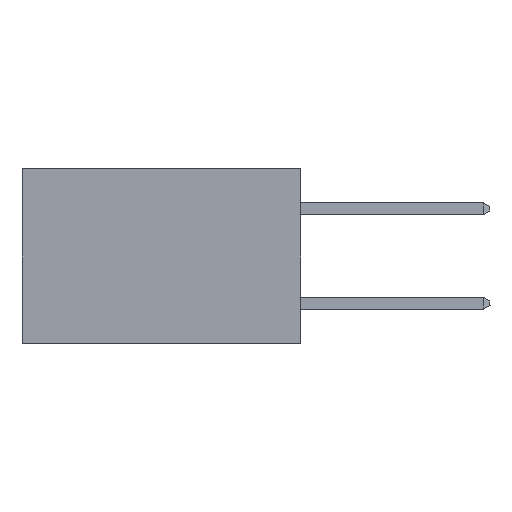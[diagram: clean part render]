
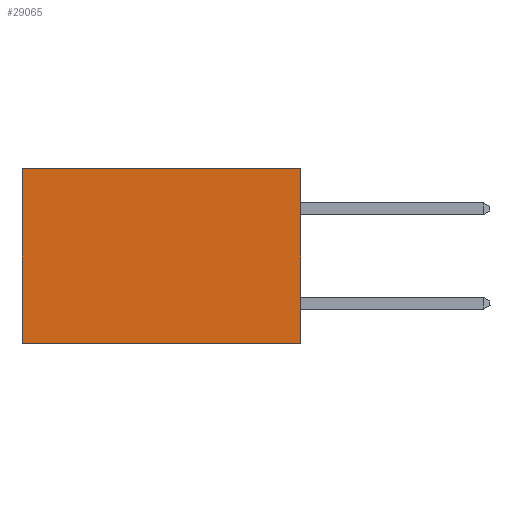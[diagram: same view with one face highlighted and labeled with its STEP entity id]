
A CAD part, left-side view. The second image highlights one B-rep face of the part: STEP entity #29065.
In plain terms, the highlighted planar face has unit normal (-1, 0, 0).
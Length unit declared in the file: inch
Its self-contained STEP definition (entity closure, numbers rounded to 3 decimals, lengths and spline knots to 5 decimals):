
#489 = EDGE_CURVE ( 'NONE', #24330, #6889, #16269, .T. ) ;
#1101 = CARTESIAN_POINT ( 'NONE',  ( 0.277, 0., -0.37 ) ) ;
#1385 = VECTOR ( 'NONE', #24439, 39.37008 ) ;
#2097 = EDGE_CURVE ( 'NONE', #6889, #4923, #13634, .T. ) ;
#4361 = ORIENTED_EDGE ( 'NONE', *, *, #17349, .T. ) ;
#4923 = VERTEX_POINT ( 'NONE', #20999 ) ;
#5316 = DIRECTION ( 'NONE',  ( 0., 1., 0. ) ) ;
#5651 = CARTESIAN_POINT ( 'NONE',  ( 0.277, 0., 0. ) ) ;
#6889 = VERTEX_POINT ( 'NONE', #11292 ) ;
#7578 = FACE_OUTER_BOUND ( 'NONE', #15338, .T. ) ;
#7612 = CARTESIAN_POINT ( 'NONE',  ( 0.277, 0., 0. ) ) ;
#8781 = VECTOR ( 'NONE', #11978, 39.37008 ) ;
#9785 = ORIENTED_EDGE ( 'NONE', *, *, #489, .F. ) ;
#10196 = VECTOR ( 'NONE', #17906, 39.37008 ) ;
#10547 = VERTEX_POINT ( 'NONE', #25921 ) ;
#11292 = CARTESIAN_POINT ( 'NONE',  ( 0.277, 0., -0.37 ) ) ;
#11978 = DIRECTION ( 'NONE',  ( 0., 0., -1. ) ) ;
#12576 = CARTESIAN_POINT ( 'NONE',  ( 0.277, 0., -0.37 ) ) ;
#13634 = LINE ( 'NONE', #12576, #1385 ) ;
#13737 = DIRECTION ( 'NONE',  ( 1., 0., 0. ) ) ;
#13950 = ORIENTED_EDGE ( 'NONE', *, *, #27455, .T. ) ;
#14354 = LINE ( 'NONE', #7612, #25838 ) ;
#14893 = LINE ( 'NONE', #23415, #8781 ) ;
#15338 = EDGE_LOOP ( 'NONE', ( #13950, #27346, #9785, #4361 ) ) ;
#16269 = LINE ( 'NONE', #1101, #10196 ) ;
#17349 = EDGE_CURVE ( 'NONE', #24330, #10547, #14354, .T. ) ;
#17906 = DIRECTION ( 'NONE',  ( 0., 0., -1. ) ) ;
#20581 = CARTESIAN_POINT ( 'NONE',  ( 0.277, 0., -0.37 ) ) ;
#20999 = CARTESIAN_POINT ( 'NONE',  ( 0.277, 0.59, -0.37 ) ) ;
#23415 = CARTESIAN_POINT ( 'NONE',  ( 0.277, 0.59, -0.37 ) ) ;
#23819 = DIRECTION ( 'NONE',  ( 0., 0., -1. ) ) ;
#24330 = VERTEX_POINT ( 'NONE', #5651 ) ;
#24439 = DIRECTION ( 'NONE',  ( 0., 1., 0. ) ) ;
#25158 = AXIS2_PLACEMENT_3D ( 'NONE', #20581, #13737, #23819 ) ;
#25838 = VECTOR ( 'NONE', #5316, 39.37008 ) ;
#25921 = CARTESIAN_POINT ( 'NONE',  ( 0.277, 0.59, 0. ) ) ;
#27346 = ORIENTED_EDGE ( 'NONE', *, *, #2097, .F. ) ;
#27455 = EDGE_CURVE ( 'NONE', #10547, #4923, #14893, .T. ) ;
#29065 = ADVANCED_FACE ( 'NONE', ( #7578 ), #29648, .F. ) ;
#29648 = PLANE ( 'NONE',  #25158 ) ;
